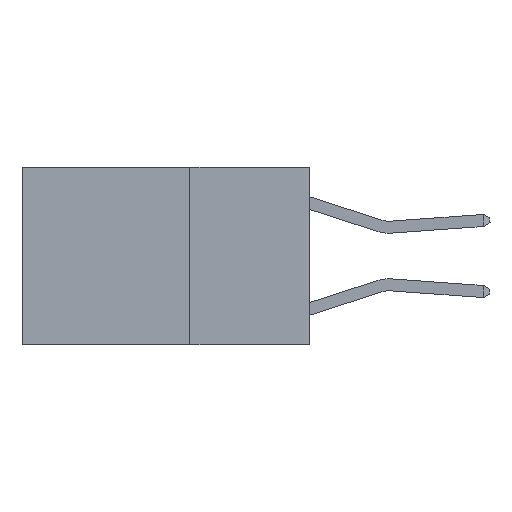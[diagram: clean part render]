
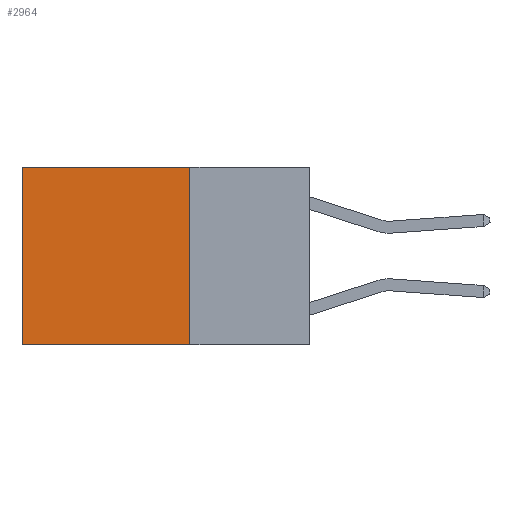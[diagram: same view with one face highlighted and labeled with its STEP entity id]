
A CAD part, left-side view. The second image highlights one B-rep face of the part: STEP entity #2964.
In plain terms, the highlighted planar face has unit normal (-1, 0, 0).
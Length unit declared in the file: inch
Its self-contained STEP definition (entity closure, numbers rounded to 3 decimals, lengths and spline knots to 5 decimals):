
#123 = ORIENTED_EDGE ( 'NONE', *, *, #5051, .T. ) ;
#318 = EDGE_CURVE ( 'NONE', #5791, #5487, #7729, .T. ) ;
#424 = DIRECTION ( 'NONE',  ( 0., 0., -1. ) ) ;
#564 = ORIENTED_EDGE ( 'NONE', *, *, #318, .F. ) ;
#1229 = CARTESIAN_POINT ( 'NONE',  ( 0.2625, 0.25, -0.37 ) ) ;
#2964 = ADVANCED_FACE ( 'NONE', ( #9902 ), #5760, .F. ) ;
#3943 = VERTEX_POINT ( 'NONE', #8885 ) ;
#4121 = CARTESIAN_POINT ( 'NONE',  ( 0.2625, 0.25, 0. ) ) ;
#4243 = ORIENTED_EDGE ( 'NONE', *, *, #5740, .T. ) ;
#4382 = CARTESIAN_POINT ( 'NONE',  ( 0.2625, 0.6, -0.37 ) ) ;
#5051 = EDGE_CURVE ( 'NONE', #3943, #7017, #9351, .T. ) ;
#5487 = VERTEX_POINT ( 'NONE', #15170 ) ;
#5740 = EDGE_CURVE ( 'NONE', #5791, #3943, #10373, .T. ) ;
#5760 = PLANE ( 'NONE',  #7107 ) ;
#5791 = VERTEX_POINT ( 'NONE', #14568 ) ;
#6168 = VECTOR ( 'NONE', #14389, 39.37008 ) ;
#6278 = EDGE_CURVE ( 'NONE', #5487, #7017, #10171, .T. ) ;
#6937 = VECTOR ( 'NONE', #13361, 39.37008 ) ;
#7017 = VERTEX_POINT ( 'NONE', #4382 ) ;
#7107 = AXIS2_PLACEMENT_3D ( 'NONE', #14884, #8255, #424 ) ;
#7487 = VECTOR ( 'NONE', #12199, 39.37008 ) ;
#7729 = LINE ( 'NONE', #14567, #13654 ) ;
#8255 = DIRECTION ( 'NONE',  ( 1., 0., 0. ) ) ;
#8885 = CARTESIAN_POINT ( 'NONE',  ( 0.2625, 0.6, 0. ) ) ;
#9351 = LINE ( 'NONE', #13290, #6168 ) ;
#9902 = FACE_OUTER_BOUND ( 'NONE', #12350, .T. ) ;
#10171 = LINE ( 'NONE', #1229, #7487 ) ;
#10234 = ORIENTED_EDGE ( 'NONE', *, *, #6278, .F. ) ;
#10373 = LINE ( 'NONE', #4121, #6937 ) ;
#12199 = DIRECTION ( 'NONE',  ( 0., 1., 0. ) ) ;
#12350 = EDGE_LOOP ( 'NONE', ( #123, #10234, #564, #4243 ) ) ;
#13290 = CARTESIAN_POINT ( 'NONE',  ( 0.2625, 0.6, 0. ) ) ;
#13361 = DIRECTION ( 'NONE',  ( 0., 1., 0. ) ) ;
#13654 = VECTOR ( 'NONE', #14522, 39.37008 ) ;
#14389 = DIRECTION ( 'NONE',  ( 0., 0., -1. ) ) ;
#14522 = DIRECTION ( 'NONE',  ( 0., 0., -1. ) ) ;
#14567 = CARTESIAN_POINT ( 'NONE',  ( 0.2625, 0.25, 0. ) ) ;
#14568 = CARTESIAN_POINT ( 'NONE',  ( 0.2625, 0.25, 0. ) ) ;
#14884 = CARTESIAN_POINT ( 'NONE',  ( 0.2625, 0.25, 0. ) ) ;
#15170 = CARTESIAN_POINT ( 'NONE',  ( 0.2625, 0.25, -0.37 ) ) ;
